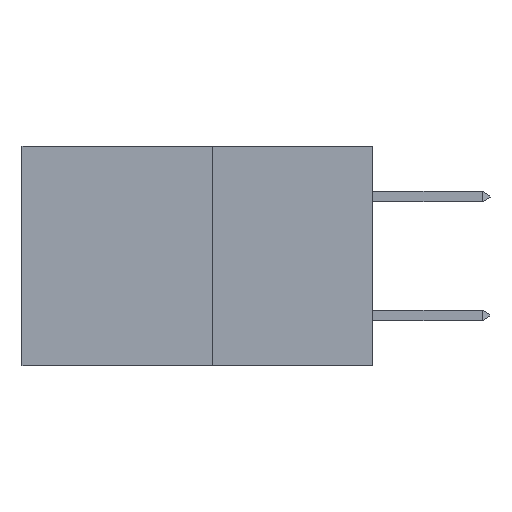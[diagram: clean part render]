
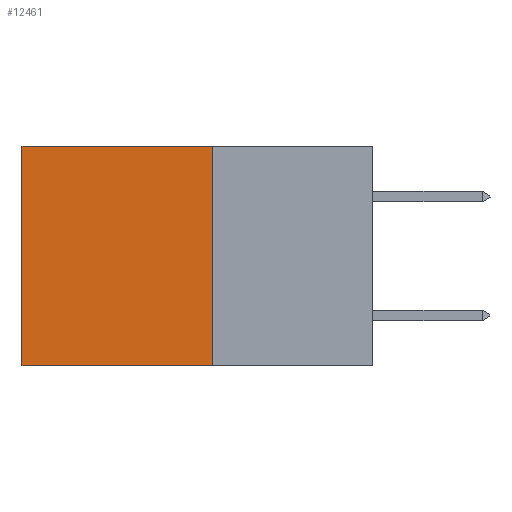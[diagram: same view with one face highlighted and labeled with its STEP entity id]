
A CAD part, left-side view. The second image highlights one B-rep face of the part: STEP entity #12461.
In plain terms, the highlighted planar face has unit normal (-1, 0, 0).
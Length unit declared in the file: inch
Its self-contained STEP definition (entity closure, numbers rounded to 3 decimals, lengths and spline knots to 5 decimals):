
#123 = VECTOR ( 'NONE', #9535, 39.37008 ) ;
#483 = LINE ( 'NONE', #11798, #123 ) ;
#1350 = VERTEX_POINT ( 'NONE', #12421 ) ;
#1533 = LINE ( 'NONE', #3614, #7240 ) ;
#2379 = CARTESIAN_POINT ( 'NONE',  ( 0.277, 0.27, 0. ) ) ;
#2626 = PLANE ( 'NONE',  #11100 ) ;
#3265 = LINE ( 'NONE', #2379, #9043 ) ;
#3578 = EDGE_CURVE ( 'NONE', #7231, #13328, #13880, .T. ) ;
#3614 = CARTESIAN_POINT ( 'NONE',  ( 0.277, 0.59, -0.37 ) ) ;
#3616 = FACE_OUTER_BOUND ( 'NONE', #6986, .T. ) ;
#4228 = CARTESIAN_POINT ( 'NONE',  ( 0.277, 0.27, -0.37 ) ) ;
#4739 = DIRECTION ( 'NONE',  ( 0., 0., -1. ) ) ;
#4987 = EDGE_CURVE ( 'NONE', #7231, #1350, #3265, .T. ) ;
#6013 = DIRECTION ( 'NONE',  ( 1., 0., 0. ) ) ;
#6808 = CARTESIAN_POINT ( 'NONE',  ( 0.277, 0.59, -0.37 ) ) ;
#6986 = EDGE_LOOP ( 'NONE', ( #14297, #13959, #14153, #11967 ) ) ;
#7085 = CARTESIAN_POINT ( 'NONE',  ( 0.277, 0.27, -0.37 ) ) ;
#7231 = VERTEX_POINT ( 'NONE', #13172 ) ;
#7240 = VECTOR ( 'NONE', #4739, 39.37008 ) ;
#7602 = VERTEX_POINT ( 'NONE', #6808 ) ;
#8072 = DIRECTION ( 'NONE',  ( 0., 1., 0. ) ) ;
#8570 = DIRECTION ( 'NONE',  ( 0., 0., -1. ) ) ;
#9043 = VECTOR ( 'NONE', #8072, 39.37008 ) ;
#9267 = EDGE_CURVE ( 'NONE', #1350, #7602, #1533, .T. ) ;
#9535 = DIRECTION ( 'NONE',  ( 0., 1., 0. ) ) ;
#10704 = CARTESIAN_POINT ( 'NONE',  ( 0.277, 0.27, -0.37 ) ) ;
#11100 = AXIS2_PLACEMENT_3D ( 'NONE', #7085, #6013, #14081 ) ;
#11798 = CARTESIAN_POINT ( 'NONE',  ( 0.277, 0.27, -0.37 ) ) ;
#11967 = ORIENTED_EDGE ( 'NONE', *, *, #4987, .T. ) ;
#12421 = CARTESIAN_POINT ( 'NONE',  ( 0.277, 0.59, 0. ) ) ;
#12461 = ADVANCED_FACE ( 'NONE', ( #3616 ), #2626, .F. ) ;
#13172 = CARTESIAN_POINT ( 'NONE',  ( 0.277, 0.27, 0. ) ) ;
#13328 = VERTEX_POINT ( 'NONE', #4228 ) ;
#13526 = VECTOR ( 'NONE', #8570, 39.37008 ) ;
#13880 = LINE ( 'NONE', #10704, #13526 ) ;
#13959 = ORIENTED_EDGE ( 'NONE', *, *, #14328, .F. ) ;
#14081 = DIRECTION ( 'NONE',  ( 0., 0., -1. ) ) ;
#14153 = ORIENTED_EDGE ( 'NONE', *, *, #3578, .F. ) ;
#14297 = ORIENTED_EDGE ( 'NONE', *, *, #9267, .T. ) ;
#14328 = EDGE_CURVE ( 'NONE', #13328, #7602, #483, .T. ) ;
